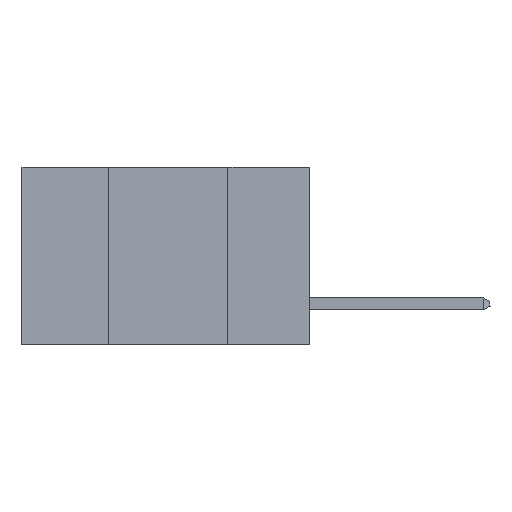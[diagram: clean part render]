
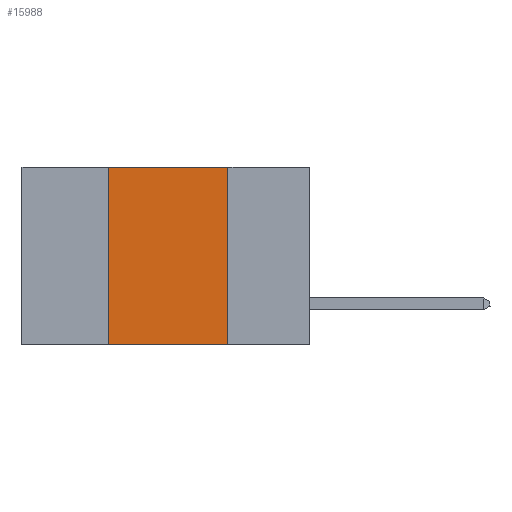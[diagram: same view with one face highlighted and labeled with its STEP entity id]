
A CAD part, left-side view. The second image highlights one B-rep face of the part: STEP entity #15988.
In plain terms, the highlighted planar face has unit normal (-1, 0, 0).
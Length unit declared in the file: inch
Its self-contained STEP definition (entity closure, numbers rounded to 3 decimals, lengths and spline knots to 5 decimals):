
#3722 = AXIS2_PLACEMENT_3D ( 'NONE', #3865, #20273, #26687 ) ;
#3865 = CARTESIAN_POINT ( 'NONE',  ( 0., 0.6, 0. ) ) ;
#4601 = ORIENTED_EDGE ( 'NONE', *, *, #30625, .F. ) ;
#5168 = VERTEX_POINT ( 'NONE', #6265 ) ;
#6265 = CARTESIAN_POINT ( 'NONE',  ( 0., 0.42, -0.37 ) ) ;
#7103 = LINE ( 'NONE', #34680, #26977 ) ;
#8207 = VECTOR ( 'NONE', #31475, 39.37008 ) ;
#8405 = CARTESIAN_POINT ( 'NONE',  ( 0., 0.17, -0.37 ) ) ;
#10773 = EDGE_CURVE ( 'NONE', #5168, #41229, #31788, .T. ) ;
#11756 = EDGE_CURVE ( 'NONE', #5168, #12630, #39374, .T. ) ;
#12495 = FACE_OUTER_BOUND ( 'NONE', #34385, .T. ) ;
#12630 = VERTEX_POINT ( 'NONE', #8405 ) ;
#15665 = CARTESIAN_POINT ( 'NONE',  ( 0., 0.6, 0. ) ) ;
#15988 = ADVANCED_FACE ( 'NONE', ( #12495 ), #39688, .F. ) ;
#19202 = EDGE_CURVE ( 'NONE', #41229, #34087, #20821, .T. ) ;
#19987 = ORIENTED_EDGE ( 'NONE', *, *, #19202, .F. ) ;
#20273 = DIRECTION ( 'NONE',  ( 1., 0., 0. ) ) ;
#20821 = LINE ( 'NONE', #15665, #28501 ) ;
#21070 = VECTOR ( 'NONE', #34804, 39.37008 ) ;
#21249 = ORIENTED_EDGE ( 'NONE', *, *, #11756, .T. ) ;
#23430 = CARTESIAN_POINT ( 'NONE',  ( 0., 0.42, 0. ) ) ;
#25660 = DIRECTION ( 'NONE',  ( 0., 0., -1. ) ) ;
#25677 = DIRECTION ( 'NONE',  ( 0., -1., 0. ) ) ;
#26687 = DIRECTION ( 'NONE',  ( 0., 0., -1. ) ) ;
#26977 = VECTOR ( 'NONE', #25660, 39.37008 ) ;
#28501 = VECTOR ( 'NONE', #25677, 39.37008 ) ;
#30625 = EDGE_CURVE ( 'NONE', #34087, #12630, #7103, .T. ) ;
#31475 = DIRECTION ( 'NONE',  ( 0., -1., 0. ) ) ;
#31788 = LINE ( 'NONE', #38479, #21070 ) ;
#31909 = CARTESIAN_POINT ( 'NONE',  ( 0., 0.6, -0.37 ) ) ;
#33453 = CARTESIAN_POINT ( 'NONE',  ( 0., 0.17, 0. ) ) ;
#34087 = VERTEX_POINT ( 'NONE', #33453 ) ;
#34385 = EDGE_LOOP ( 'NONE', ( #4601, #19987, #34572, #21249 ) ) ;
#34572 = ORIENTED_EDGE ( 'NONE', *, *, #10773, .F. ) ;
#34680 = CARTESIAN_POINT ( 'NONE',  ( 0., 0.17, 0. ) ) ;
#34804 = DIRECTION ( 'NONE',  ( 0., 0., 1. ) ) ;
#38479 = CARTESIAN_POINT ( 'NONE',  ( 0., 0.42, 0. ) ) ;
#39374 = LINE ( 'NONE', #31909, #8207 ) ;
#39688 = PLANE ( 'NONE',  #3722 ) ;
#41229 = VERTEX_POINT ( 'NONE', #23430 ) ;
